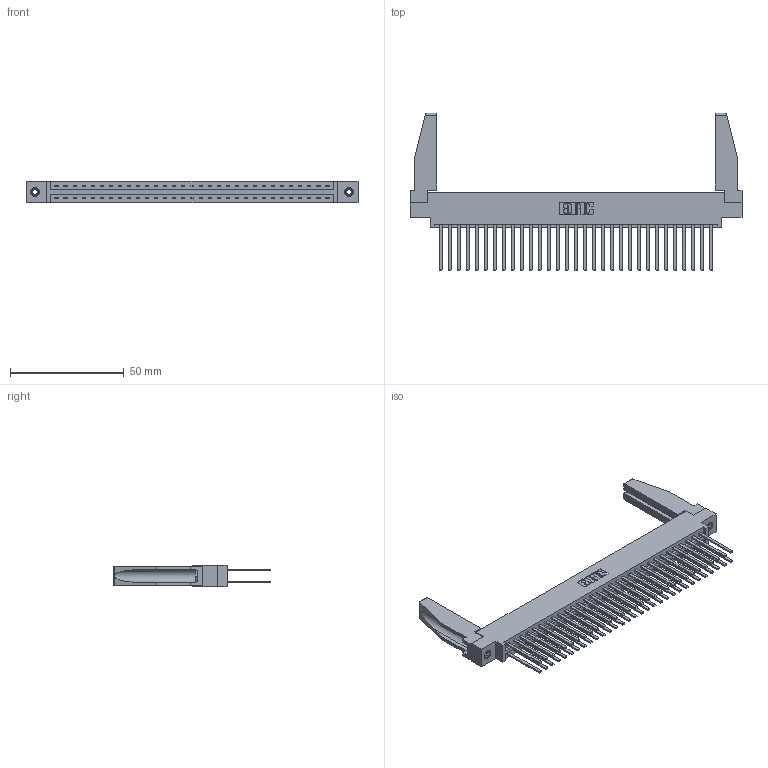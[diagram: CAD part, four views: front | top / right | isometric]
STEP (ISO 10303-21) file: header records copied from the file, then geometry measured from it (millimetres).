
FILE_DESCRIPTION (( 'STEP AP203' ), '1' );
FILE_NAME ('387-062-544-878.STEP', '2019-10-19T15:24:27', ( '' ), ( '' ), 'SwSTEP 2.0', 'SolidWorks 2016', '' );
FILE_SCHEMA (( 'CONFIG_CONTROL_DESIGN' ));
Length unit declared in the file: inch
Products named in the file (5): 345-250-001_345-250-001-102; 387-062-544-878; 337 Part_0.170 Offset - 0.156 Dia-TI; 307-220-078; 345-292-001_345-293-144
Assembly tree (67 placements, depth 2):
  387-062-544-878
    337 Part_0.170 Offset - 0.156 Dia-TI
    345-292-001_345-293-144  x62
    345-250-001_345-250-001-102  x2
    307-220-078  x2
Bounding box: 145.85 x 69.09 x 9.4 mm (x, y, z)
Volume: 19969 mm3; surface area: 24731.2 mm2
Topology: 67 solids, 67 shells, 3224 faces, 9519 edges, 6254 vertices
Faces by surface type: plane 2266, cylinder 942, cone 12, torus 4
Entity records: 27846 total; most frequent: CARTESIAN_POINT 4700, ORIENTED_EDGE 4592, DIRECTION 4020, EDGE_CURVE 2296, LINE 2134, VECTOR 2134, VERTEX_POINT 1524, AXIS2_PLACEMENT_3D 943
